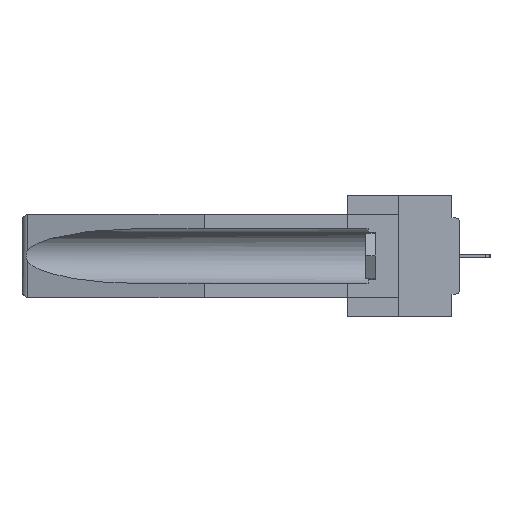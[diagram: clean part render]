
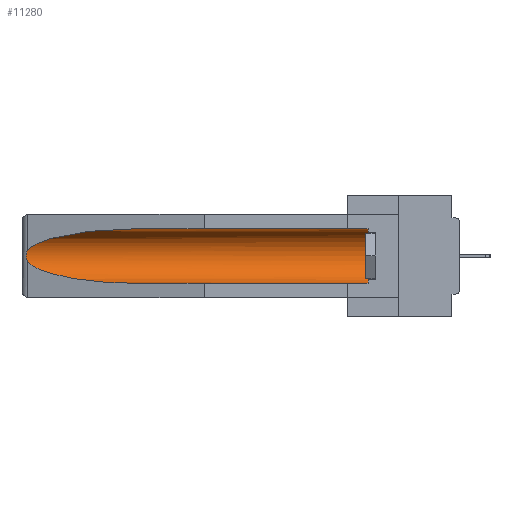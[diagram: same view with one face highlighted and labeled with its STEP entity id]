
A CAD part, left-side view. The second image highlights one B-rep face of the part: STEP entity #11280.
In plain terms, the highlighted cylindrical face has radius 2.857 mm (diameter 5.715 mm), a partial arc.
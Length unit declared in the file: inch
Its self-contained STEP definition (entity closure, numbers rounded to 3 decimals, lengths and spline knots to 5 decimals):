
#189 = CARTESIAN_POINT ( 'NONE',  ( 0.155, -0.30754, -0.059 ) ) ;
#405 = DIRECTION ( 'NONE',  ( 0., 1., 0. ) ) ;
#804 = EDGE_CURVE ( 'NONE', #17143, #26745, #19085, .T. ) ;
#1185 = CARTESIAN_POINT ( 'NONE',  ( 0.155, 1.07973, -0.059 ) ) ;
#1802 = CARTESIAN_POINT ( 'NONE',  ( 0.2673, 1.5327, -0.16383 ) ) ;
#1981 = CARTESIAN_POINT ( 'NONE',  ( 0.26537, 1.52718, -0.19328 ) ) ;
#4164 = CARTESIAN_POINT ( 'NONE',  ( 0.155, 1.07973, -0.059 ) ) ;
#4215 = CARTESIAN_POINT ( 'NONE',  ( 0.26537, 1.52718, -0.14972 ) ) ;
#4730 = EDGE_CURVE ( 'NONE', #26745, #34439, #19657, .T. ) ;
#5105 = CARTESIAN_POINT ( 'NONE',  ( 0.155, 0.126, -0.059 ) ) ;
#5832 = CARTESIAN_POINT ( 'NONE',  ( 0.155, 0.126, -0.284 ) ) ;
#6659 = DIRECTION ( 'NONE',  ( 0., -1., 0. ) ) ;
#7501 = CARTESIAN_POINT ( 'NONE',  ( 0.26654, 1.53092, -0.15636 ) ) ;
#7666 = ORIENTED_EDGE ( 'NONE', *, *, #4730, .T. ) ;
#9567 = CARTESIAN_POINT ( 'NONE',  ( 0.21114, 1.30732, -0.059 ) ) ;
#9910 = ORIENTED_EDGE ( 'NONE', *, *, #804, .T. ) ;
#10189 = CARTESIAN_POINT ( 'NONE',  ( 0.2673, 1.53269, -0.17917 ) ) ;
#11280 = ADVANCED_FACE ( 'NONE', ( #31759 ), #25873, .F. ) ;
#11797 = CARTESIAN_POINT ( 'NONE',  ( 0.155, -0.30754, -0.1715 ) ) ;
#11892 = DIRECTION ( 'NONE',  ( 0., 1., 0. ) ) ;
#13580 = CARTESIAN_POINT ( 'NONE',  ( 0.26597, 1.5296, -0.19026 ) ) ;
#14420 = AXIS2_PLACEMENT_3D ( 'NONE', #11797, #405, #34999 ) ;
#15042 = EDGE_CURVE ( 'NONE', #22519, #34439, #29574, .T. ) ;
#15072 = CARTESIAN_POINT ( 'NONE',  ( 0.26537, 1.52718, -0.19328 ) ) ;
#15504 = VERTEX_POINT ( 'NONE', #5105 ) ;
#15886 = CARTESIAN_POINT ( 'NONE',  ( 0.26655, 1.53094, -0.18657 ) ) ;
#16333 = EDGE_LOOP ( 'NONE', ( #27173, #9910, #7666, #29217, #21260, #34271 ) ) ;
#16929 = CARTESIAN_POINT ( 'NONE',  ( 0.26537, 1.52718, -0.19328 ) ) ;
#17143 = VERTEX_POINT ( 'NONE', #29667 ) ;
#17848 = LINE ( 'NONE', #189, #31186 ) ;
#18453 = CARTESIAN_POINT ( 'NONE',  ( 0.25451, 1.48313, -0.09465 ) ) ;
#19085 = B_SPLINE_CURVE_WITH_KNOTS ( 'NONE', 3,
 ( #24971, #33541, #7501, #1802, #36401, #22322, #10189, #15886, #13580, #1981 ),
 .UNSPECIFIED., .F., .F.,
 ( 4, 2, 2, 2, 4 ),
 ( 0., 0.00029, 0.00058, 0.00087, 0.00117 ),
 .UNSPECIFIED. ) ;
#19657 =( BOUNDED_CURVE ( )  B_SPLINE_CURVE ( 3, ( #15072, #23757, #29682, #23585 ),
 .UNSPECIFIED., .F., .F. ) 
 B_SPLINE_CURVE_WITH_KNOTS ( ( 4, 4 ),
 ( 0.1948, 1.5708 ),
 .UNSPECIFIED. ) 
 CURVE ( )  GEOMETRIC_REPRESENTATION_ITEM ( )  RATIONAL_B_SPLINE_CURVE ( ( 1., 0.848, 0.848, 1. ) ) 
 REPRESENTATION_ITEM ( '' )  );
#19982 = AXIS2_PLACEMENT_3D ( 'NONE', #35915, #6659, #26984 ) ;
#21260 = ORIENTED_EDGE ( 'NONE', *, *, #30065, .T. ) ;
#22322 = CARTESIAN_POINT ( 'NONE',  ( 0.2675, 1.53308, -0.17534 ) ) ;
#22519 = VERTEX_POINT ( 'NONE', #5832 ) ;
#23585 = CARTESIAN_POINT ( 'NONE',  ( 0.155, 1.07973, -0.284 ) ) ;
#23660 = CIRCLE ( 'NONE', #19982, 0.1125 ) ;
#23757 = CARTESIAN_POINT ( 'NONE',  ( 0.25451, 1.48313, -0.24835 ) ) ;
#24971 = CARTESIAN_POINT ( 'NONE',  ( 0.26537, 1.52718, -0.14972 ) ) ;
#25873 = CYLINDRICAL_SURFACE ( 'NONE', #14420, 0.1125 ) ;
#26745 = VERTEX_POINT ( 'NONE', #16929 ) ;
#26882 = CARTESIAN_POINT ( 'NONE',  ( 0.155, -0.30754, -0.284 ) ) ;
#26984 = DIRECTION ( 'NONE',  ( 0., 0., 1. ) ) ;
#27173 = ORIENTED_EDGE ( 'NONE', *, *, #29645, .T. ) ;
#29093 = DIRECTION ( 'NONE',  ( 0., 1., 0. ) ) ;
#29217 = ORIENTED_EDGE ( 'NONE', *, *, #15042, .F. ) ;
#29574 = LINE ( 'NONE', #26882, #33733 ) ;
#29645 = EDGE_CURVE ( 'NONE', #35785, #17143, #33016, .T. ) ;
#29667 = CARTESIAN_POINT ( 'NONE',  ( 0.26537, 1.52718, -0.14972 ) ) ;
#29682 = CARTESIAN_POINT ( 'NONE',  ( 0.21114, 1.30732, -0.284 ) ) ;
#30065 = EDGE_CURVE ( 'NONE', #22519, #15504, #23660, .T. ) ;
#31186 = VECTOR ( 'NONE', #29093, 39.37008 ) ;
#31759 = FACE_OUTER_BOUND ( 'NONE', #16333, .T. ) ;
#33016 =( BOUNDED_CURVE ( )  B_SPLINE_CURVE ( 3, ( #1185, #9567, #18453, #4215 ),
 .UNSPECIFIED., .F., .F. ) 
 B_SPLINE_CURVE_WITH_KNOTS ( ( 4, 4 ),
 ( 4.71239, 6.08839 ),
 .UNSPECIFIED. ) 
 CURVE ( )  GEOMETRIC_REPRESENTATION_ITEM ( )  RATIONAL_B_SPLINE_CURVE ( ( 1., 0.848, 0.848, 1. ) ) 
 REPRESENTATION_ITEM ( '' )  );
#33541 = CARTESIAN_POINT ( 'NONE',  ( 0.26597, 1.52961, -0.15275 ) ) ;
#33733 = VECTOR ( 'NONE', #11892, 39.37008 ) ;
#34271 = ORIENTED_EDGE ( 'NONE', *, *, #36934, .T. ) ;
#34439 = VERTEX_POINT ( 'NONE', #34915 ) ;
#34915 = CARTESIAN_POINT ( 'NONE',  ( 0.155, 1.07973, -0.284 ) ) ;
#34999 = DIRECTION ( 'NONE',  ( 0., 0., 1. ) ) ;
#35785 = VERTEX_POINT ( 'NONE', #4164 ) ;
#35915 = CARTESIAN_POINT ( 'NONE',  ( 0.155, 0.126, -0.1715 ) ) ;
#36401 = CARTESIAN_POINT ( 'NONE',  ( 0.2675, 1.53308, -0.16763 ) ) ;
#36934 = EDGE_CURVE ( 'NONE', #15504, #35785, #17848, .T. ) ;
